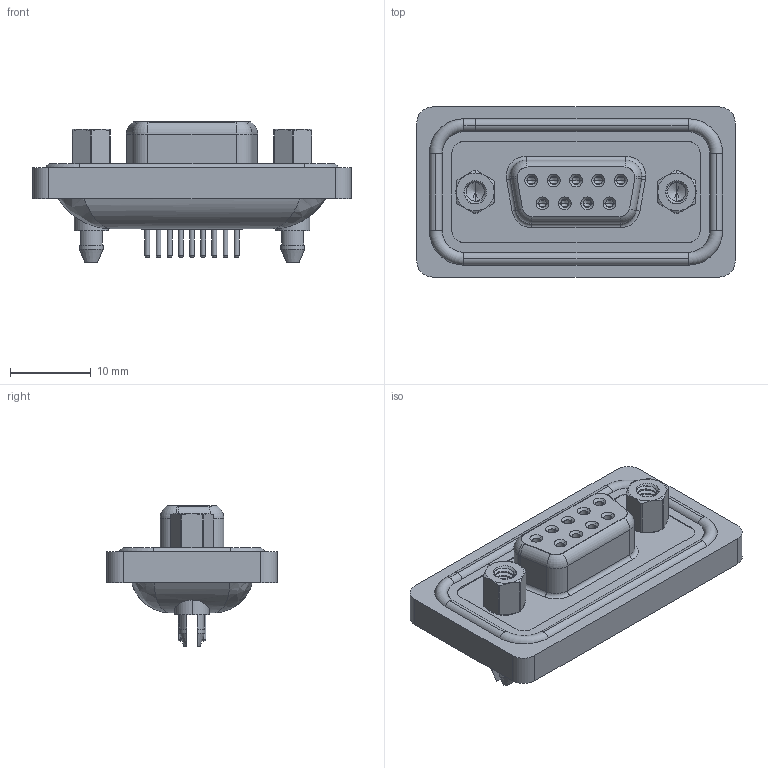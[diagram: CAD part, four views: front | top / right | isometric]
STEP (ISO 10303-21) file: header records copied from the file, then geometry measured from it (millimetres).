
FILE_DESCRIPTION (( 'STEP AP203' ), '1' );
FILE_NAME ('628-W09-220-013.STEP', '2021-04-06T14:25:53', ( '' ), ( '' ), 'SwSTEP 2.0', 'SolidWorks 2020', '' );
FILE_SCHEMA (( 'CONFIG_CONTROL_DESIGN' ));
Length unit declared in the file: millimetre
Products named in the file (8): 628W Housing_09 Contacts; 628W 4-40 Hex Standoff; 628-W09-220-013; 628W Waterproof Housing_09 Contacts BL; 628W Contact Row 2_20; 628W Contact Row 1_20; 628W Shell Front_09 Contacts; 628W 4-40 Threaded Boardlock
Assembly tree (16 placements, depth 2):
  628-W09-220-013
    628W Housing_09 Contacts
    628W Shell Front_09 Contacts
    628W Contact Row 1_20  x5
    628W Contact Row 2_20  x4
    628W 4-40 Threaded Boardlock  x2
    628W Waterproof Housing_09 Contacts BL
    628W 4-40 Hex Standoff  x2
Bounding box: 39.5 x 21.1 x 17.45 mm (x, y, z)
Volume: 5093.2 mm3; surface area: 7764.1 mm2
Topology: 17 solids, 17 shells, 984 faces, 2406 edges, 1505 vertices
Faces by surface type: cylinder 441, plane 250, torus 176, cone 95, bspline 22
Entity records: 22120 total; most frequent: CARTESIAN_POINT 7530, DIRECTION 2966, ORIENTED_EDGE 2774, EDGE_CURVE 1387, AXIS2_PLACEMENT_3D 1221, VERTEX_POINT 885, EDGE_LOOP 666, CIRCLE 647
